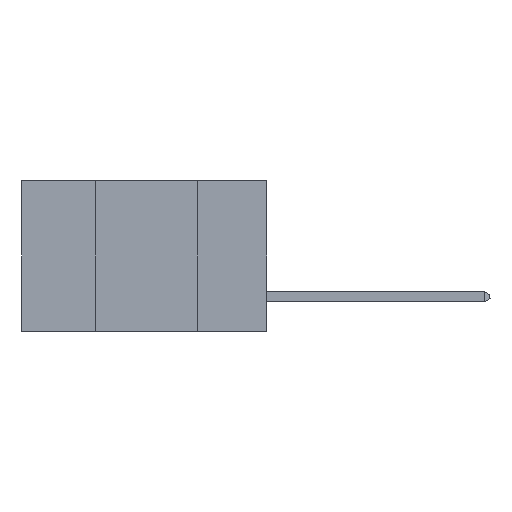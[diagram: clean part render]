
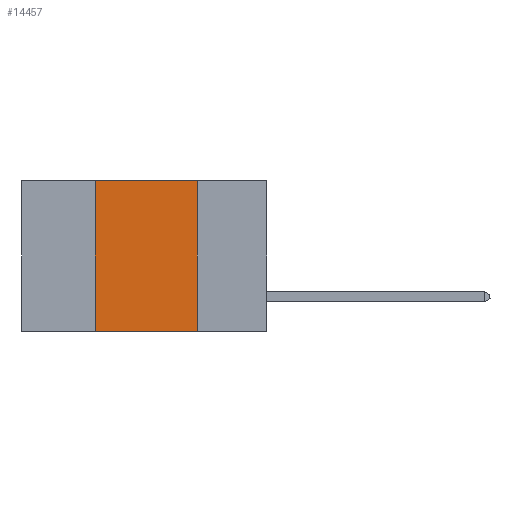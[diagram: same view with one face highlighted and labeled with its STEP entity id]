
A CAD part, left-side view. The second image highlights one B-rep face of the part: STEP entity #14457.
In plain terms, the highlighted planar face has unit normal (-1, 0, 0).
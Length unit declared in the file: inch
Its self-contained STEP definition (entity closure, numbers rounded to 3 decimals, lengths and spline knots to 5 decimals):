
#583 = LINE ( 'NONE', #17133, #6929 ) ;
#749 = LINE ( 'NONE', #14322, #1214 ) ;
#1214 = VECTOR ( 'NONE', #14255, 39.37008 ) ;
#1751 = LINE ( 'NONE', #15005, #9672 ) ;
#2231 = CARTESIAN_POINT ( 'NONE',  ( 0., 0.6, 0. ) ) ;
#2362 = ORIENTED_EDGE ( 'NONE', *, *, #10337, .F. ) ;
#2772 = EDGE_LOOP ( 'NONE', ( #2362, #15633, #4312, #10852 ) ) ;
#3712 = LINE ( 'NONE', #4951, #16092 ) ;
#4312 = ORIENTED_EDGE ( 'NONE', *, *, #9596, .F. ) ;
#4915 = CARTESIAN_POINT ( 'NONE',  ( 0., 0.17, 0. ) ) ;
#4951 = CARTESIAN_POINT ( 'NONE',  ( 0., 0.6, 0. ) ) ;
#5227 = CARTESIAN_POINT ( 'NONE',  ( 0., 0.42, -0.37 ) ) ;
#5789 = FACE_OUTER_BOUND ( 'NONE', #2772, .T. ) ;
#6929 = VECTOR ( 'NONE', #18557, 39.37008 ) ;
#7135 = VERTEX_POINT ( 'NONE', #4915 ) ;
#7545 = EDGE_CURVE ( 'NONE', #16402, #17878, #583, .T. ) ;
#9596 = EDGE_CURVE ( 'NONE', #16402, #13667, #1751, .T. ) ;
#9672 = VECTOR ( 'NONE', #11939, 39.37008 ) ;
#10337 = EDGE_CURVE ( 'NONE', #7135, #17878, #749, .T. ) ;
#10493 = PLANE ( 'NONE',  #13246 ) ;
#10761 = CARTESIAN_POINT ( 'NONE',  ( 0., 0.42, 0. ) ) ;
#10852 = ORIENTED_EDGE ( 'NONE', *, *, #7545, .T. ) ;
#10924 = DIRECTION ( 'NONE',  ( 0., -1., 0. ) ) ;
#11000 = DIRECTION ( 'NONE',  ( 0., 0., -1. ) ) ;
#11063 = DIRECTION ( 'NONE',  ( 1., 0., 0. ) ) ;
#11939 = DIRECTION ( 'NONE',  ( 0., 0., 1. ) ) ;
#13085 = EDGE_CURVE ( 'NONE', #13667, #7135, #3712, .T. ) ;
#13246 = AXIS2_PLACEMENT_3D ( 'NONE', #2231, #11063, #11000 ) ;
#13667 = VERTEX_POINT ( 'NONE', #10761 ) ;
#14255 = DIRECTION ( 'NONE',  ( 0., 0., -1. ) ) ;
#14322 = CARTESIAN_POINT ( 'NONE',  ( 0., 0.17, 0. ) ) ;
#14457 = ADVANCED_FACE ( 'NONE', ( #5789 ), #10493, .F. ) ;
#15005 = CARTESIAN_POINT ( 'NONE',  ( 0., 0.42, 0. ) ) ;
#15522 = CARTESIAN_POINT ( 'NONE',  ( 0., 0.17, -0.37 ) ) ;
#15633 = ORIENTED_EDGE ( 'NONE', *, *, #13085, .F. ) ;
#16092 = VECTOR ( 'NONE', #10924, 39.37008 ) ;
#16402 = VERTEX_POINT ( 'NONE', #5227 ) ;
#17133 = CARTESIAN_POINT ( 'NONE',  ( 0., 0.6, -0.37 ) ) ;
#17878 = VERTEX_POINT ( 'NONE', #15522 ) ;
#18557 = DIRECTION ( 'NONE',  ( 0., -1., 0. ) ) ;
